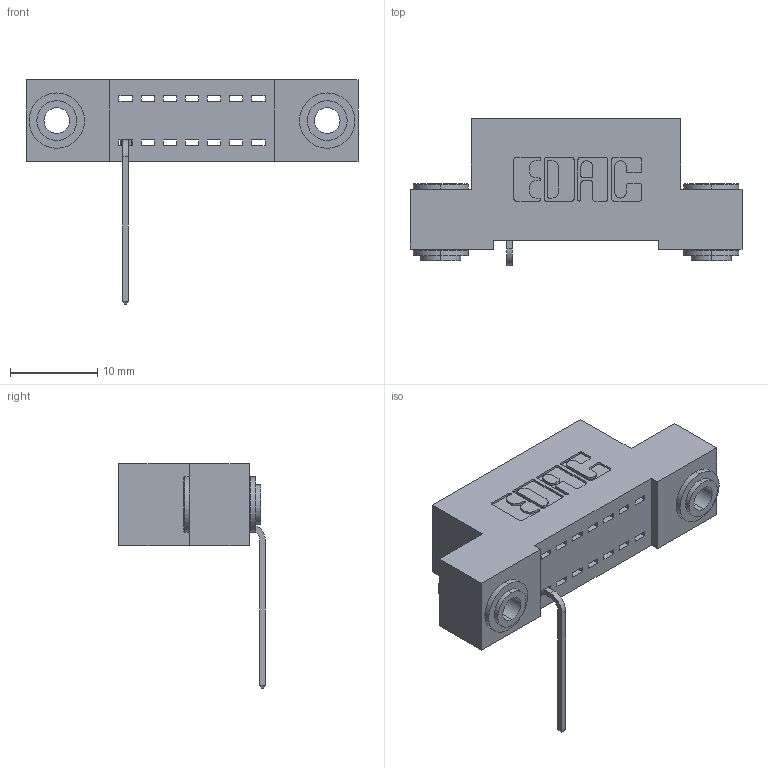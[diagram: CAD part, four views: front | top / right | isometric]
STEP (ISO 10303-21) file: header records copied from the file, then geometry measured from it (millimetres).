
FILE_DESCRIPTION (( 'STEP AP203' ), '1' );
FILE_NAME ('392-007-559-103.STEP', '2018-08-14T19:04:31', ( '' ), ( '' ), 'SwSTEP 2.0', 'SolidWorks 2016', '' );
FILE_SCHEMA (( 'CONFIG_CONTROL_DESIGN' ));
Length unit declared in the file: inch
Products named in the file (4): 345-292-001_558 559 Tail - 1; 342-250-002_345-250-002-102; 392-007-559-103; 342 Part_.156 TH
Assembly tree (4 placements, depth 2):
  392-007-559-103
    342 Part_.156 TH
    345-292-001_558 559 Tail - 1
    342-250-002_345-250-002-102  x2
Bounding box: 38.1 x 16.83 x 25.78 mm (x, y, z)
Volume: 3169.2 mm3; surface area: 3889.9 mm2
Topology: 4 solids, 4 shells, 280 faces, 809 edges, 534 vertices
Faces by surface type: plane 192, cylinder 80, cone 8
Entity records: 9216 total; most frequent: CARTESIAN_POINT 1600, ORIENTED_EDGE 1542, DIRECTION 1447, EDGE_CURVE 771, VECTOR 619, LINE 619, VERTEX_POINT 510, AXIS2_PLACEMENT_3D 414
